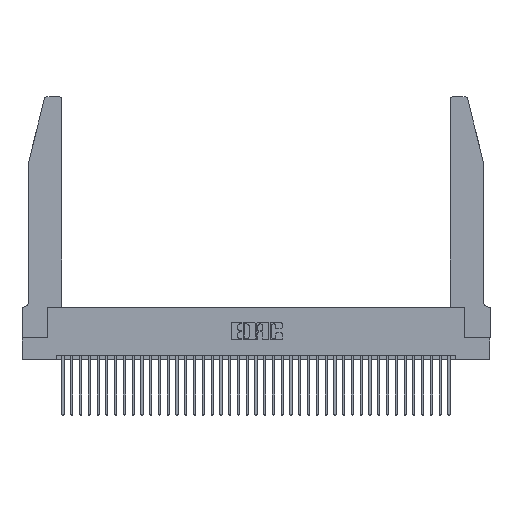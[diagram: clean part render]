
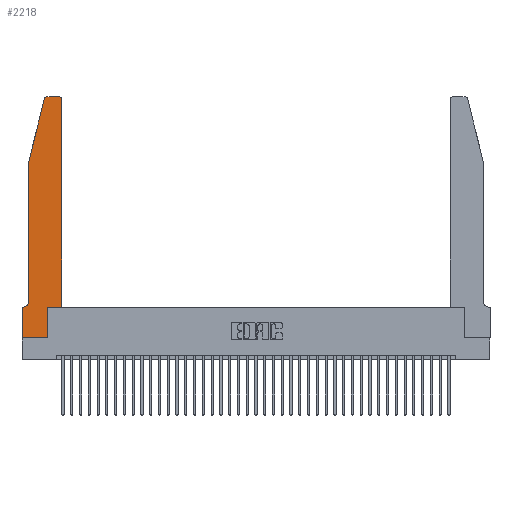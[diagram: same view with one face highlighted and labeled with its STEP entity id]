
A CAD part, top view. The second image highlights one B-rep face of the part: STEP entity #2218.
In plain terms, the highlighted planar face has unit normal (0, 0, 1).
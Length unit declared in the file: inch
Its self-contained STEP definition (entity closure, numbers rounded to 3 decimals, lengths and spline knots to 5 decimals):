
#354 = ORIENTED_EDGE ( 'NONE', *, *, #10784, .T. ) ;
#1611 = ORIENTED_EDGE ( 'NONE', *, *, #4649, .T. ) ;
#1906 = EDGE_LOOP ( 'NONE', ( #28506, #16730, #36942, #1611, #354, #29247, #35166, #26851, #27779, #26191, #15164, #20253 ) ) ;
#1947 = LINE ( 'NONE', #10678, #3857 ) ;
#2184 = AXIS2_PLACEMENT_3D ( 'NONE', #14438, #39087, #36111 ) ;
#2218 = ADVANCED_FACE ( 'NONE', ( #22386 ), #33980, .T. ) ;
#2245 = EDGE_CURVE ( 'NONE', #19885, #28363, #21938, .T. ) ;
#2376 = EDGE_CURVE ( 'NONE', #28363, #3091, #12801, .T. ) ;
#2400 = DIRECTION ( 'NONE',  ( 1., 0., 0. ) ) ;
#2532 = LINE ( 'NONE', #22419, #37501 ) ;
#3091 = VERTEX_POINT ( 'NONE', #18794 ) ;
#3425 = DIRECTION ( 'NONE',  ( -1., 0., 0. ) ) ;
#3837 = CARTESIAN_POINT ( 'NONE',  ( 0.4505, 0.35, 0.37 ) ) ;
#3857 = VECTOR ( 'NONE', #16994, 39.37008 ) ;
#4018 = LINE ( 'NONE', #3837, #5515 ) ;
#4610 = VECTOR ( 'NONE', #7619, 39.37008 ) ;
#4649 = EDGE_CURVE ( 'NONE', #14652, #9407, #28886, .T. ) ;
#4724 = DIRECTION ( 'NONE',  ( -1., 0., 0. ) ) ;
#5504 = AXIS2_PLACEMENT_3D ( 'NONE', #10781, #23126, #4724 ) ;
#5515 = VECTOR ( 'NONE', #10296, 39.37008 ) ;
#5608 = CARTESIAN_POINT ( 'NONE',  ( 0.4205, 2.72, 0.37 ) ) ;
#6036 = VERTEX_POINT ( 'NONE', #12071 ) ;
#7619 = DIRECTION ( 'NONE',  ( 0., -1., 0. ) ) ;
#7740 = VERTEX_POINT ( 'NONE', #32868 ) ;
#8696 = DIRECTION ( 'NONE',  ( 0., 0., 1. ) ) ;
#9407 = VERTEX_POINT ( 'NONE', #15470 ) ;
#9789 = CIRCLE ( 'NONE', #2184, 0.03 ) ;
#10296 = DIRECTION ( 'NONE',  ( 0., 1., 0. ) ) ;
#10678 = CARTESIAN_POINT ( 'NONE',  ( 0.0755, 2., 0.37 ) ) ;
#10781 = CARTESIAN_POINT ( 'NONE',  ( 0.0055, 0.42, 0.37 ) ) ;
#10784 = EDGE_CURVE ( 'NONE', #9407, #19885, #38565, .T. ) ;
#11091 = DIRECTION ( 'NONE',  ( 0., 1., 0. ) ) ;
#11948 = EDGE_CURVE ( 'NONE', #36284, #7740, #2532, .T. ) ;
#11957 = CARTESIAN_POINT ( 'NONE',  ( 0.2865, 0.35, 0.37 ) ) ;
#12071 = CARTESIAN_POINT ( 'NONE',  ( 0.4205, 2.75, 0.37 ) ) ;
#12291 = CARTESIAN_POINT ( 'NONE',  ( 0., 0.35, 0.37 ) ) ;
#12698 = VERTEX_POINT ( 'NONE', #17587 ) ;
#12801 = LINE ( 'NONE', #25734, #4610 ) ;
#12957 = DIRECTION ( 'NONE',  ( 0., 0., 1. ) ) ;
#13141 = CARTESIAN_POINT ( 'NONE',  ( 0.0055, 0.35, 0.37 ) ) ;
#13166 = AXIS2_PLACEMENT_3D ( 'NONE', #5608, #8696, #2400 ) ;
#13521 = LINE ( 'NONE', #23450, #34612 ) ;
#13702 = EDGE_CURVE ( 'NONE', #29011, #14652, #1947, .T. ) ;
#14438 = CARTESIAN_POINT ( 'NONE',  ( 0.284, 2.72, 0.37 ) ) ;
#14652 = VERTEX_POINT ( 'NONE', #22112 ) ;
#15164 = ORIENTED_EDGE ( 'NONE', *, *, #37053, .T. ) ;
#15470 = CARTESIAN_POINT ( 'NONE',  ( 0.0755, 0.42, 0.37 ) ) ;
#16730 = ORIENTED_EDGE ( 'NONE', *, *, #37388, .T. ) ;
#16994 = DIRECTION ( 'NONE',  ( -0.239, -0.971, 0. ) ) ;
#17370 = LINE ( 'NONE', #32619, #24052 ) ;
#17587 = CARTESIAN_POINT ( 'NONE',  ( 0.4505, 2.72, 0.37 ) ) ;
#18794 = CARTESIAN_POINT ( 'NONE',  ( 0., 0., 0.37 ) ) ;
#18874 = CARTESIAN_POINT ( 'NONE',  ( 0., 0.35, 0.37 ) ) ;
#18986 = VERTEX_POINT ( 'NONE', #28734 ) ;
#19885 = VERTEX_POINT ( 'NONE', #13141 ) ;
#20253 = ORIENTED_EDGE ( 'NONE', *, *, #33786, .T. ) ;
#21264 = LINE ( 'NONE', #24367, #29829 ) ;
#21938 = LINE ( 'NONE', #34232, #29080 ) ;
#22112 = CARTESIAN_POINT ( 'NONE',  ( 0.0755, 2., 0.37 ) ) ;
#22386 = FACE_OUTER_BOUND ( 'NONE', #1906, .T. ) ;
#22419 = CARTESIAN_POINT ( 'NONE',  ( 0.4505, 0.35, 0.37 ) ) ;
#23126 = DIRECTION ( 'NONE',  ( 0., 0., -1. ) ) ;
#23300 = CARTESIAN_POINT ( 'NONE',  ( 0.0755, 2., 0.37 ) ) ;
#23309 = VERTEX_POINT ( 'NONE', #30499 ) ;
#23450 = CARTESIAN_POINT ( 'NONE',  ( 0., 0., 0.37 ) ) ;
#24052 = VECTOR ( 'NONE', #11091, 39.37008 ) ;
#24229 = DIRECTION ( 'NONE',  ( -1., 0., 0. ) ) ;
#24367 = CARTESIAN_POINT ( 'NONE',  ( 0.2605, 2.75, 0.37 ) ) ;
#24762 = DIRECTION ( 'NONE',  ( 1., 0., 0. ) ) ;
#24972 = EDGE_CURVE ( 'NONE', #18986, #36284, #17370, .T. ) ;
#25734 = CARTESIAN_POINT ( 'NONE',  ( 0., 0., 0.37 ) ) ;
#26191 = ORIENTED_EDGE ( 'NONE', *, *, #11948, .T. ) ;
#26523 = DIRECTION ( 'NONE',  ( 1., 0., 0. ) ) ;
#26851 = ORIENTED_EDGE ( 'NONE', *, *, #28193, .T. ) ;
#27779 = ORIENTED_EDGE ( 'NONE', *, *, #24972, .T. ) ;
#28193 = EDGE_CURVE ( 'NONE', #3091, #18986, #13521, .T. ) ;
#28340 = EDGE_CURVE ( 'NONE', #6036, #23309, #21264, .T. ) ;
#28363 = VERTEX_POINT ( 'NONE', #12291 ) ;
#28506 = ORIENTED_EDGE ( 'NONE', *, *, #28340, .T. ) ;
#28734 = CARTESIAN_POINT ( 'NONE',  ( 0.2865, 0., 0.37 ) ) ;
#28886 = LINE ( 'NONE', #23300, #29388 ) ;
#29011 = VERTEX_POINT ( 'NONE', #30580 ) ;
#29080 = VECTOR ( 'NONE', #3425, 39.37008 ) ;
#29247 = ORIENTED_EDGE ( 'NONE', *, *, #2245, .T. ) ;
#29388 = VECTOR ( 'NONE', #38823, 39.37008 ) ;
#29829 = VECTOR ( 'NONE', #24229, 39.37008 ) ;
#30499 = CARTESIAN_POINT ( 'NONE',  ( 0.284, 2.75, 0.37 ) ) ;
#30580 = CARTESIAN_POINT ( 'NONE',  ( 0.25487, 2.72718, 0.37 ) ) ;
#32619 = CARTESIAN_POINT ( 'NONE',  ( 0.2865, 0.35, 0.37 ) ) ;
#32868 = CARTESIAN_POINT ( 'NONE',  ( 0.4505, 0.35, 0.37 ) ) ;
#33786 = EDGE_CURVE ( 'NONE', #12698, #6036, #39042, .T. ) ;
#33980 = PLANE ( 'NONE',  #37745 ) ;
#34232 = CARTESIAN_POINT ( 'NONE',  ( 0.0755, 0.35, 0.37 ) ) ;
#34612 = VECTOR ( 'NONE', #26523, 39.37008 ) ;
#35166 = ORIENTED_EDGE ( 'NONE', *, *, #2376, .T. ) ;
#36111 = DIRECTION ( 'NONE',  ( 1., 0., 0. ) ) ;
#36284 = VERTEX_POINT ( 'NONE', #11957 ) ;
#36942 = ORIENTED_EDGE ( 'NONE', *, *, #13702, .T. ) ;
#37053 = EDGE_CURVE ( 'NONE', #7740, #12698, #4018, .T. ) ;
#37388 = EDGE_CURVE ( 'NONE', #23309, #29011, #9789, .T. ) ;
#37501 = VECTOR ( 'NONE', #39290, 39.37008 ) ;
#37745 = AXIS2_PLACEMENT_3D ( 'NONE', #18874, #12957, #24762 ) ;
#38565 = CIRCLE ( 'NONE', #5504, 0.07 ) ;
#38823 = DIRECTION ( 'NONE',  ( 0., -1., 0. ) ) ;
#39042 = CIRCLE ( 'NONE', #13166, 0.03 ) ;
#39087 = DIRECTION ( 'NONE',  ( 0., 0., 1. ) ) ;
#39290 = DIRECTION ( 'NONE',  ( 1., 0., 0. ) ) ;
